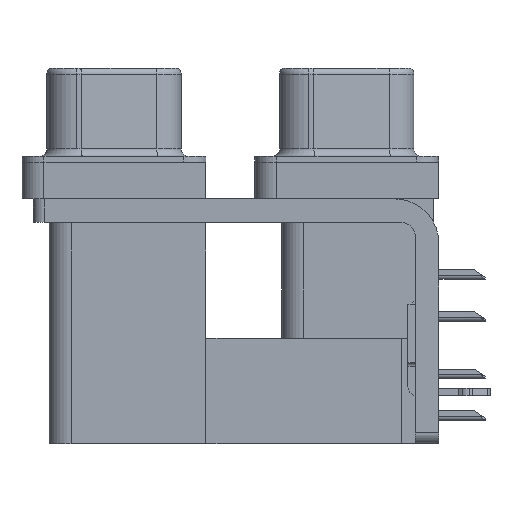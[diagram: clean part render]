
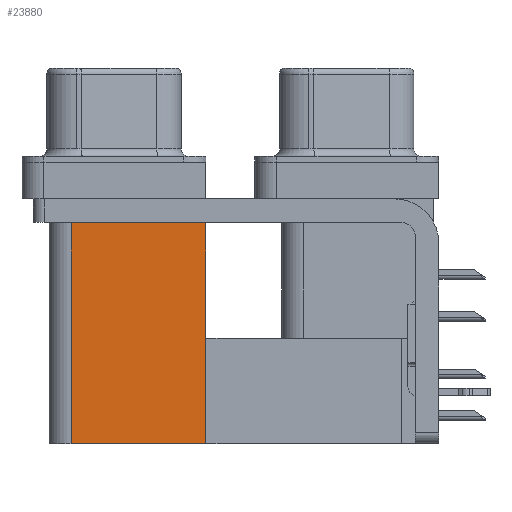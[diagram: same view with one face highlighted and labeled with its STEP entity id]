
A CAD part, left-side view. The second image highlights one B-rep face of the part: STEP entity #23880.
In plain terms, the highlighted planar face has unit normal (-1, 0, 0).
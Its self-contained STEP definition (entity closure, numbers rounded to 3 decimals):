
#1174 = EDGE_LOOP ( 'NONE', ( #26162, #26410, #26544, #7281 ) ) ;
#1690 = VECTOR ( 'NONE', #29981, 1000. ) ;
#2263 = CARTESIAN_POINT ( 'NONE',  ( 3.765, 9.6, -19.2 ) ) ;
#5545 = CARTESIAN_POINT ( 'NONE',  ( 3.765, 18.8, -19.2 ) ) ;
#5697 = LINE ( 'NONE', #5545, #6756 ) ;
#6756 = VECTOR ( 'NONE', #22066, 1000. ) ;
#7281 = ORIENTED_EDGE ( 'NONE', *, *, #30607, .T. ) ;
#8727 = VECTOR ( 'NONE', #25832, 1000. ) ;
#8748 = DIRECTION ( 'NONE',  ( 1., 0., 0. ) ) ;
#9206 = DIRECTION ( 'NONE',  ( 0., 0., -1. ) ) ;
#9251 = CARTESIAN_POINT ( 'NONE',  ( 3.765, 9.6, -2.5 ) ) ;
#9294 = LINE ( 'NONE', #2263, #8727 ) ;
#10351 = VERTEX_POINT ( 'NONE', #21643 ) ;
#12245 = VERTEX_POINT ( 'NONE', #27764 ) ;
#13268 = VERTEX_POINT ( 'NONE', #9251 ) ;
#13288 = LINE ( 'NONE', #22803, #1690 ) ;
#13571 = FACE_OUTER_BOUND ( 'NONE', #1174, .T. ) ;
#13896 = PLANE ( 'NONE',  #21200 ) ;
#14101 = EDGE_CURVE ( 'NONE', #10351, #29367, #9294, .T. ) ;
#14264 = EDGE_CURVE ( 'NONE', #29367, #12245, #5697, .T. ) ;
#15105 = DIRECTION ( 'NONE',  ( 0., 0., 1. ) ) ;
#15574 = CARTESIAN_POINT ( 'NONE',  ( 3.765, 9.6, -19.2 ) ) ;
#18935 = CARTESIAN_POINT ( 'NONE',  ( 3.765, 18.8, -19.2 ) ) ;
#21200 = AXIS2_PLACEMENT_3D ( 'NONE', #23389, #8748, #9206 ) ;
#21643 = CARTESIAN_POINT ( 'NONE',  ( 3.765, 9.6, -19.2 ) ) ;
#22066 = DIRECTION ( 'NONE',  ( 0., 0., 1. ) ) ;
#22734 = LINE ( 'NONE', #15574, #30087 ) ;
#22803 = CARTESIAN_POINT ( 'NONE',  ( 3.765, 9.6, -2.5 ) ) ;
#23389 = CARTESIAN_POINT ( 'NONE',  ( 3.765, 9.6, -19.2 ) ) ;
#23880 = ADVANCED_FACE ( 'NONE', ( #13571 ), #13896, .F. ) ;
#25832 = DIRECTION ( 'NONE',  ( 0., 1., 0. ) ) ;
#26162 = ORIENTED_EDGE ( 'NONE', *, *, #28350, .T. ) ;
#26410 = ORIENTED_EDGE ( 'NONE', *, *, #14264, .F. ) ;
#26544 = ORIENTED_EDGE ( 'NONE', *, *, #14101, .F. ) ;
#27764 = CARTESIAN_POINT ( 'NONE',  ( 3.765, 18.8, -2.5 ) ) ;
#28350 = EDGE_CURVE ( 'NONE', #13268, #12245, #13288, .T. ) ;
#29367 = VERTEX_POINT ( 'NONE', #18935 ) ;
#29981 = DIRECTION ( 'NONE',  ( 0., 1., 0. ) ) ;
#30087 = VECTOR ( 'NONE', #15105, 1000. ) ;
#30607 = EDGE_CURVE ( 'NONE', #10351, #13268, #22734, .T. ) ;
